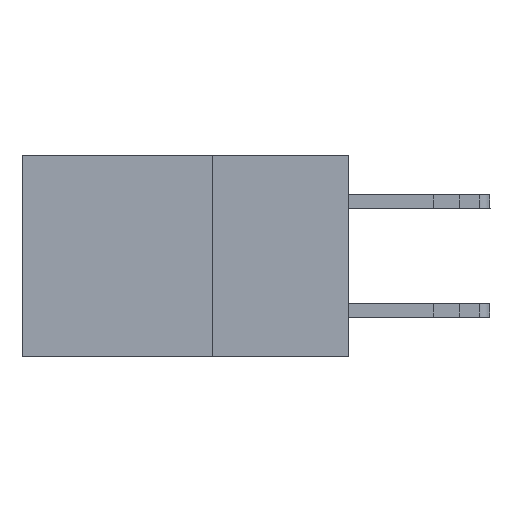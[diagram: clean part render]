
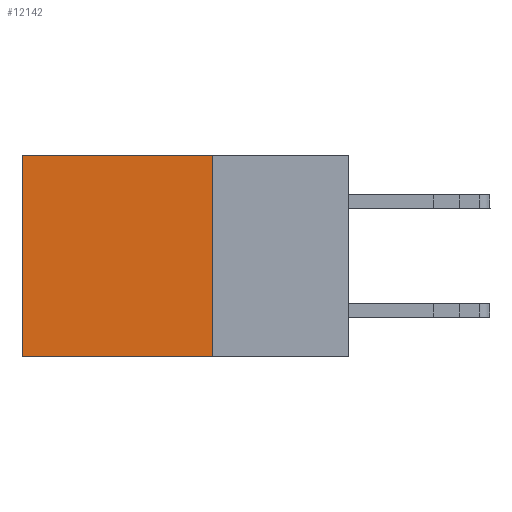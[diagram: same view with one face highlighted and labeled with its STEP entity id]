
A CAD part, left-side view. The second image highlights one B-rep face of the part: STEP entity #12142.
In plain terms, the highlighted planar face has unit normal (-1, 0, 0).
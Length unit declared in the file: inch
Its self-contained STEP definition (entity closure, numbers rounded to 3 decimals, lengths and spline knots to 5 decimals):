
#574 = LINE ( 'NONE', #16902, #5046 ) ;
#1120 = CARTESIAN_POINT ( 'NONE',  ( 0.298, 0.25, 0. ) ) ;
#1356 = EDGE_CURVE ( 'NONE', #4674, #1538, #13728, .T. ) ;
#1521 = VECTOR ( 'NONE', #12479, 39.37008 ) ;
#1538 = VERTEX_POINT ( 'NONE', #14383 ) ;
#2239 = DIRECTION ( 'NONE',  ( 0., 0., -1. ) ) ;
#3024 = CARTESIAN_POINT ( 'NONE',  ( 0.298, 0.25, -0.37 ) ) ;
#4136 = AXIS2_PLACEMENT_3D ( 'NONE', #10561, #12213, #2239 ) ;
#4674 = VERTEX_POINT ( 'NONE', #3024 ) ;
#5046 = VECTOR ( 'NONE', #7062, 39.37008 ) ;
#5900 = EDGE_CURVE ( 'NONE', #19733, #1538, #574, .T. ) ;
#7062 = DIRECTION ( 'NONE',  ( 0., 0., -1. ) ) ;
#7782 = CARTESIAN_POINT ( 'NONE',  ( 0.298, 0.25, 0. ) ) ;
#7793 = VECTOR ( 'NONE', #17647, 39.37008 ) ;
#9364 = VECTOR ( 'NONE', #19700, 39.37008 ) ;
#10561 = CARTESIAN_POINT ( 'NONE',  ( 0.298, 0.25, 0. ) ) ;
#10797 = CARTESIAN_POINT ( 'NONE',  ( 0.298, 0.6, 0. ) ) ;
#11379 = VERTEX_POINT ( 'NONE', #7782 ) ;
#12142 = ADVANCED_FACE ( 'NONE', ( #14694 ), #20401, .F. ) ;
#12213 = DIRECTION ( 'NONE',  ( 1., 0., 0. ) ) ;
#12479 = DIRECTION ( 'NONE',  ( 0., 0., -1. ) ) ;
#12974 = EDGE_CURVE ( 'NONE', #11379, #4674, #18607, .T. ) ;
#13086 = EDGE_CURVE ( 'NONE', #11379, #19733, #20927, .T. ) ;
#13728 = LINE ( 'NONE', #20606, #9364 ) ;
#13943 = ORIENTED_EDGE ( 'NONE', *, *, #5900, .T. ) ;
#14198 = CARTESIAN_POINT ( 'NONE',  ( 0.298, 0.25, 0. ) ) ;
#14383 = CARTESIAN_POINT ( 'NONE',  ( 0.298, 0.6, -0.37 ) ) ;
#14694 = FACE_OUTER_BOUND ( 'NONE', #19235, .T. ) ;
#14981 = ORIENTED_EDGE ( 'NONE', *, *, #12974, .F. ) ;
#16150 = ORIENTED_EDGE ( 'NONE', *, *, #13086, .T. ) ;
#16651 = ORIENTED_EDGE ( 'NONE', *, *, #1356, .F. ) ;
#16902 = CARTESIAN_POINT ( 'NONE',  ( 0.298, 0.6, 0. ) ) ;
#17647 = DIRECTION ( 'NONE',  ( 0., 1., 0. ) ) ;
#18607 = LINE ( 'NONE', #14198, #1521 ) ;
#19235 = EDGE_LOOP ( 'NONE', ( #13943, #16651, #14981, #16150 ) ) ;
#19700 = DIRECTION ( 'NONE',  ( 0., 1., 0. ) ) ;
#19733 = VERTEX_POINT ( 'NONE', #10797 ) ;
#20401 = PLANE ( 'NONE',  #4136 ) ;
#20606 = CARTESIAN_POINT ( 'NONE',  ( 0.298, 0.25, -0.37 ) ) ;
#20927 = LINE ( 'NONE', #1120, #7793 ) ;
